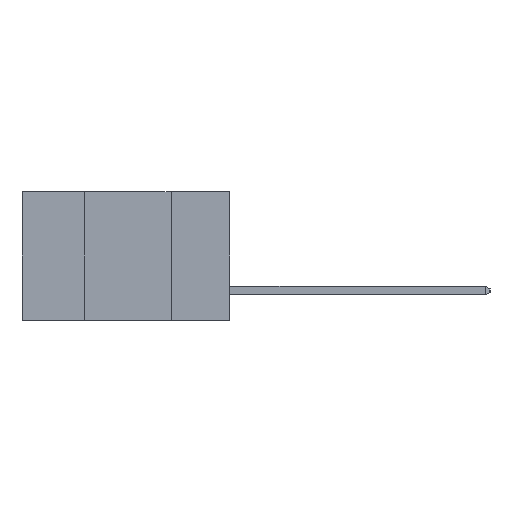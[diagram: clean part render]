
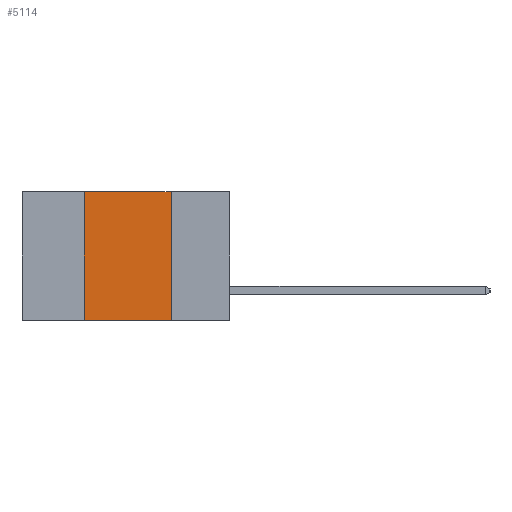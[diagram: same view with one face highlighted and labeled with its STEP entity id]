
A CAD part, left-side view. The second image highlights one B-rep face of the part: STEP entity #5114.
In plain terms, the highlighted planar face has unit normal (-1, 0, 0).
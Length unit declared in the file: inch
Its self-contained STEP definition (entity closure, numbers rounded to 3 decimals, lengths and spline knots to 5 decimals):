
#10 = ORIENTED_EDGE ( 'NONE', *, *, #6827, .F. ) ;
#181 = CARTESIAN_POINT ( 'NONE',  ( 0., 0.42, -0.37 ) ) ;
#219 = AXIS2_PLACEMENT_3D ( 'NONE', #2378, #3174, #8540 ) ;
#908 = DIRECTION ( 'NONE',  ( 0., 0., -1. ) ) ;
#1118 = EDGE_CURVE ( 'NONE', #9943, #8783, #7508, .T. ) ;
#1423 = VECTOR ( 'NONE', #4506, 39.37008 ) ;
#1975 = CARTESIAN_POINT ( 'NONE',  ( 0., 0.17, -0.37 ) ) ;
#2177 = VERTEX_POINT ( 'NONE', #9219 ) ;
#2378 = CARTESIAN_POINT ( 'NONE',  ( 0., 0.6, 0. ) ) ;
#2381 = ORIENTED_EDGE ( 'NONE', *, *, #4194, .F. ) ;
#3174 = DIRECTION ( 'NONE',  ( 1., 0., 0. ) ) ;
#3280 = VECTOR ( 'NONE', #3604, 39.37008 ) ;
#3604 = DIRECTION ( 'NONE',  ( 0., 0., 1. ) ) ;
#4194 = EDGE_CURVE ( 'NONE', #4263, #2177, #5520, .T. ) ;
#4223 = CARTESIAN_POINT ( 'NONE',  ( 0., 0.6, 0. ) ) ;
#4263 = VERTEX_POINT ( 'NONE', #4492 ) ;
#4449 = ORIENTED_EDGE ( 'NONE', *, *, #7006, .F. ) ;
#4492 = CARTESIAN_POINT ( 'NONE',  ( 0., 0.42, 0. ) ) ;
#4506 = DIRECTION ( 'NONE',  ( 0., -1., 0. ) ) ;
#4717 = DIRECTION ( 'NONE',  ( 0., -1., 0. ) ) ;
#4975 = CARTESIAN_POINT ( 'NONE',  ( 0., 0.17, -0.37 ) ) ;
#4981 = VECTOR ( 'NONE', #908, 39.37008 ) ;
#5114 = ADVANCED_FACE ( 'NONE', ( #5264 ), #7810, .F. ) ;
#5264 = FACE_OUTER_BOUND ( 'NONE', #9829, .T. ) ;
#5520 = LINE ( 'NONE', #4223, #8598 ) ;
#5599 = LINE ( 'NONE', #8973, #3280 ) ;
#6532 = ORIENTED_EDGE ( 'NONE', *, *, #1118, .T. ) ;
#6827 = EDGE_CURVE ( 'NONE', #2177, #8783, #7048, .T. ) ;
#7006 = EDGE_CURVE ( 'NONE', #9943, #4263, #5599, .T. ) ;
#7048 = LINE ( 'NONE', #4975, #4981 ) ;
#7508 = LINE ( 'NONE', #7842, #1423 ) ;
#7810 = PLANE ( 'NONE',  #219 ) ;
#7842 = CARTESIAN_POINT ( 'NONE',  ( 0., 0.6, -0.37 ) ) ;
#8540 = DIRECTION ( 'NONE',  ( 0., 0., -1. ) ) ;
#8598 = VECTOR ( 'NONE', #4717, 39.37008 ) ;
#8783 = VERTEX_POINT ( 'NONE', #1975 ) ;
#8973 = CARTESIAN_POINT ( 'NONE',  ( 0., 0.42, -0.37 ) ) ;
#9219 = CARTESIAN_POINT ( 'NONE',  ( 0., 0.17, 0. ) ) ;
#9829 = EDGE_LOOP ( 'NONE', ( #10, #2381, #4449, #6532 ) ) ;
#9943 = VERTEX_POINT ( 'NONE', #181 ) ;
